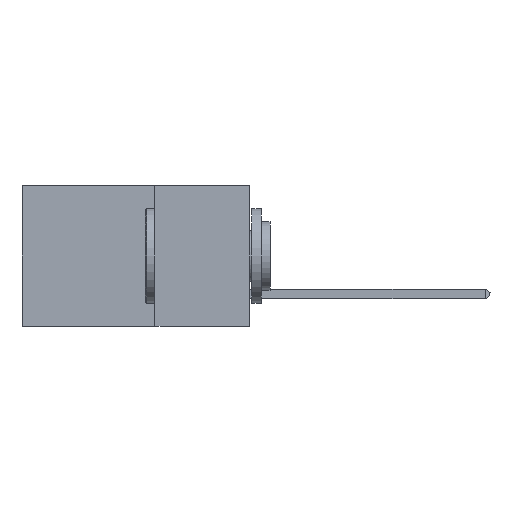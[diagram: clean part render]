
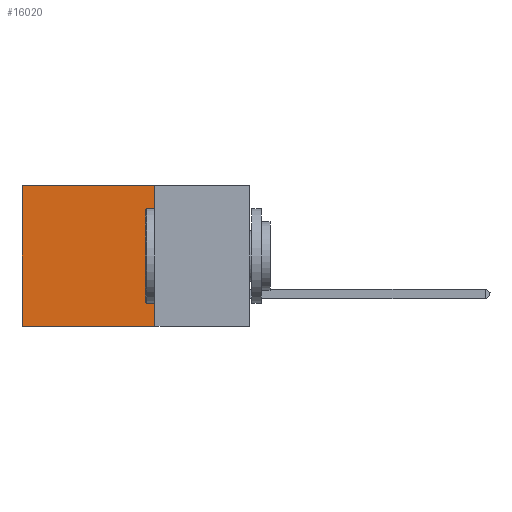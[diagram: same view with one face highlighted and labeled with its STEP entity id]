
A CAD part, left-side view. The second image highlights one B-rep face of the part: STEP entity #16020.
In plain terms, the highlighted planar face has unit normal (-1, 0, 0).
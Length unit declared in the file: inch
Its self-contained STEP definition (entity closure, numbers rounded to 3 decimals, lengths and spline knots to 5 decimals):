
#764 = VERTEX_POINT ( 'NONE', #12794 ) ;
#1337 = EDGE_CURVE ( 'NONE', #17624, #764, #27801, .T. ) ;
#1905 = VERTEX_POINT ( 'NONE', #37070 ) ;
#1983 = CARTESIAN_POINT ( 'NONE',  ( 0.2875, 0.25, -0.37 ) ) ;
#2315 = FACE_OUTER_BOUND ( 'NONE', #10329, .T. ) ;
#3564 = VECTOR ( 'NONE', #24190, 39.37008 ) ;
#3901 = CARTESIAN_POINT ( 'NONE',  ( 0.2875, 0.25, 0. ) ) ;
#6301 = VERTEX_POINT ( 'NONE', #7868 ) ;
#7868 = CARTESIAN_POINT ( 'NONE',  ( 0.2875, 0.25, 0. ) ) ;
#8015 = AXIS2_PLACEMENT_3D ( 'NONE', #3901, #29981, #28359 ) ;
#9810 = PLANE ( 'NONE',  #8015 ) ;
#10329 = EDGE_LOOP ( 'NONE', ( #32975, #32345, #30317, #31123 ) ) ;
#12145 = CARTESIAN_POINT ( 'NONE',  ( 0.2875, 0.25, 0. ) ) ;
#12773 = EDGE_CURVE ( 'NONE', #1905, #764, #28698, .T. ) ;
#12794 = CARTESIAN_POINT ( 'NONE',  ( 0.2875, 0.6, -0.37 ) ) ;
#16020 = ADVANCED_FACE ( 'NONE', ( #2315 ), #9810, .F. ) ;
#16830 = EDGE_CURVE ( 'NONE', #6301, #1905, #31410, .T. ) ;
#17624 = VERTEX_POINT ( 'NONE', #22411 ) ;
#20028 = DIRECTION ( 'NONE',  ( 0., 0., -1. ) ) ;
#22411 = CARTESIAN_POINT ( 'NONE',  ( 0.2875, 0.6, 0. ) ) ;
#24190 = DIRECTION ( 'NONE',  ( 0., 0., -1. ) ) ;
#24669 = LINE ( 'NONE', #12145, #30933 ) ;
#24677 = DIRECTION ( 'NONE',  ( 0., 1., 0. ) ) ;
#27801 = LINE ( 'NONE', #28584, #30496 ) ;
#28359 = DIRECTION ( 'NONE',  ( 0., 0., -1. ) ) ;
#28563 = EDGE_CURVE ( 'NONE', #6301, #17624, #24669, .T. ) ;
#28584 = CARTESIAN_POINT ( 'NONE',  ( 0.2875, 0.6, 0. ) ) ;
#28698 = LINE ( 'NONE', #1983, #34990 ) ;
#29981 = DIRECTION ( 'NONE',  ( 1., 0., 0. ) ) ;
#30096 = CARTESIAN_POINT ( 'NONE',  ( 0.2875, 0.25, 0. ) ) ;
#30317 = ORIENTED_EDGE ( 'NONE', *, *, #16830, .F. ) ;
#30496 = VECTOR ( 'NONE', #20028, 39.37008 ) ;
#30933 = VECTOR ( 'NONE', #31406, 39.37008 ) ;
#31123 = ORIENTED_EDGE ( 'NONE', *, *, #28563, .T. ) ;
#31406 = DIRECTION ( 'NONE',  ( 0., 1., 0. ) ) ;
#31410 = LINE ( 'NONE', #30096, #3564 ) ;
#32345 = ORIENTED_EDGE ( 'NONE', *, *, #12773, .F. ) ;
#32975 = ORIENTED_EDGE ( 'NONE', *, *, #1337, .T. ) ;
#34990 = VECTOR ( 'NONE', #24677, 39.37008 ) ;
#37070 = CARTESIAN_POINT ( 'NONE',  ( 0.2875, 0.25, -0.37 ) ) ;
